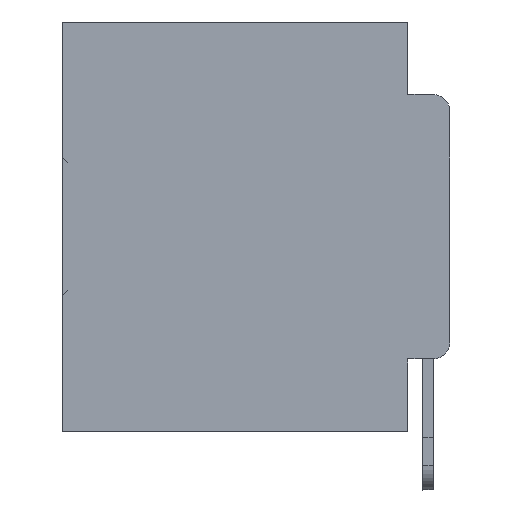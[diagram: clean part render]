
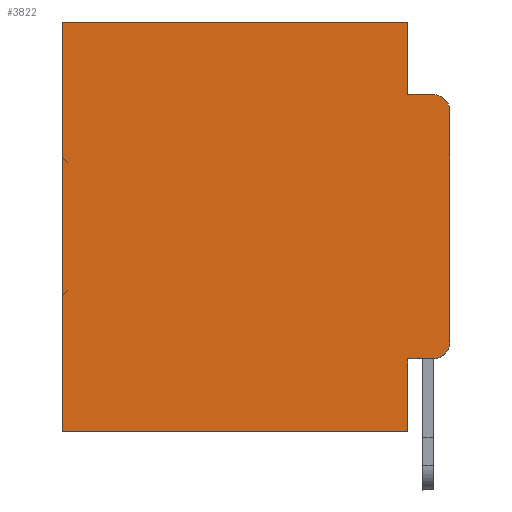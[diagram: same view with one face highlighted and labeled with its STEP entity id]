
A CAD part, left-side view. The second image highlights one B-rep face of the part: STEP entity #3822.
In plain terms, the highlighted planar face has unit normal (-1, 0, 0).
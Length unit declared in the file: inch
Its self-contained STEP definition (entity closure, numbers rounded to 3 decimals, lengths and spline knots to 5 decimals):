
#352 = VERTEX_POINT ( 'NONE', #25775 ) ;
#742 = ORIENTED_EDGE ( 'NONE', *, *, #15955, .T. ) ;
#1709 = EDGE_CURVE ( 'NONE', #17315, #6882, #31972, .T. ) ;
#2109 = FACE_OUTER_BOUND ( 'NONE', #27719, .T. ) ;
#2655 = CARTESIAN_POINT ( 'NONE',  ( 0.298, 0.051, -0.0885 ) ) ;
#2982 = DIRECTION ( 'NONE',  ( 0., 1., 0. ) ) ;
#3738 = EDGE_CURVE ( 'NONE', #15102, #352, #27232, .T. ) ;
#3822 = ADVANCED_FACE ( 'NONE', ( #2109 ), #8404, .F. ) ;
#3905 = LINE ( 'NONE', #7316, #31118 ) ;
#4172 = VERTEX_POINT ( 'NONE', #20966 ) ;
#4477 = CARTESIAN_POINT ( 'NONE',  ( 0.298, 0.02, -0.1085 ) ) ;
#4622 = CARTESIAN_POINT ( 'NONE',  ( 0.298, 0.473, 0. ) ) ;
#4858 = LINE ( 'NONE', #4622, #24842 ) ;
#5087 = CARTESIAN_POINT ( 'NONE',  ( 0.298, 0.02, -0.4115 ) ) ;
#6058 = LINE ( 'NONE', #23870, #23077 ) ;
#6618 = CARTESIAN_POINT ( 'NONE',  ( 0.298, 0.051, -0.0885 ) ) ;
#6882 = VERTEX_POINT ( 'NONE', #34267 ) ;
#6976 = EDGE_CURVE ( 'NONE', #32671, #15608, #25471, .T. ) ;
#7316 = CARTESIAN_POINT ( 'NONE',  ( 0.298, 0.051, 0. ) ) ;
#7762 = LINE ( 'NONE', #33624, #21792 ) ;
#8161 = ORIENTED_EDGE ( 'NONE', *, *, #6976, .T. ) ;
#8404 = PLANE ( 'NONE',  #27809 ) ;
#8769 = VERTEX_POINT ( 'NONE', #34031 ) ;
#9169 = ORIENTED_EDGE ( 'NONE', *, *, #22297, .F. ) ;
#9246 = DIRECTION ( 'NONE',  ( 0., -1., 0. ) ) ;
#9436 = CARTESIAN_POINT ( 'NONE',  ( 0.298, 0., -0.1085 ) ) ;
#10993 = CARTESIAN_POINT ( 'NONE',  ( 0.298, 0.051, -0.5 ) ) ;
#11136 = DIRECTION ( 'NONE',  ( 1., 0., 0. ) ) ;
#11978 = LINE ( 'NONE', #13156, #23455 ) ;
#12300 = ORIENTED_EDGE ( 'NONE', *, *, #1709, .T. ) ;
#12671 = VERTEX_POINT ( 'NONE', #10993 ) ;
#13156 = CARTESIAN_POINT ( 'NONE',  ( 0.298, 0., 0. ) ) ;
#13269 = ORIENTED_EDGE ( 'NONE', *, *, #22045, .T. ) ;
#13586 = CARTESIAN_POINT ( 'NONE',  ( 0.298, 0., -0.5 ) ) ;
#13804 = CARTESIAN_POINT ( 'NONE',  ( 0.298, 0.051, 0. ) ) ;
#15102 = VERTEX_POINT ( 'NONE', #5087 ) ;
#15574 = DIRECTION ( 'NONE',  ( 0., 0., -1. ) ) ;
#15599 = AXIS2_PLACEMENT_3D ( 'NONE', #4477, #23486, #26235 ) ;
#15608 = VERTEX_POINT ( 'NONE', #20099 ) ;
#15955 = EDGE_CURVE ( 'NONE', #6882, #4172, #4858, .T. ) ;
#16057 = LINE ( 'NONE', #6618, #27477 ) ;
#16277 = DIRECTION ( 'NONE',  ( 0., 0., -1. ) ) ;
#16452 = AXIS2_PLACEMENT_3D ( 'NONE', #32266, #24303, #16277 ) ;
#17315 = VERTEX_POINT ( 'NONE', #13804 ) ;
#17327 = DIRECTION ( 'NONE',  ( 0., 1., 0. ) ) ;
#20099 = CARTESIAN_POINT ( 'NONE',  ( 0.298, 0.02, -0.0885 ) ) ;
#20966 = CARTESIAN_POINT ( 'NONE',  ( 0.298, 0.473, -0.5 ) ) ;
#21792 = VECTOR ( 'NONE', #28279, 39.37008 ) ;
#22045 = EDGE_CURVE ( 'NONE', #8769, #15102, #7762, .T. ) ;
#22258 = ORIENTED_EDGE ( 'NONE', *, *, #3738, .T. ) ;
#22297 = EDGE_CURVE ( 'NONE', #8769, #12671, #6058, .T. ) ;
#22422 = DIRECTION ( 'NONE',  ( 0., 0., -1. ) ) ;
#22916 = EDGE_CURVE ( 'NONE', #32671, #352, #11978, .T. ) ;
#23077 = VECTOR ( 'NONE', #34887, 39.37008 ) ;
#23455 = VECTOR ( 'NONE', #32130, 39.37008 ) ;
#23486 = DIRECTION ( 'NONE',  ( -1., 0., 0. ) ) ;
#23870 = CARTESIAN_POINT ( 'NONE',  ( 0.298, 0.051, 0. ) ) ;
#23881 = LINE ( 'NONE', #13586, #31106 ) ;
#24303 = DIRECTION ( 'NONE',  ( -1., 0., 0. ) ) ;
#24517 = ORIENTED_EDGE ( 'NONE', *, *, #22916, .F. ) ;
#24570 = EDGE_CURVE ( 'NONE', #12671, #4172, #23881, .T. ) ;
#24842 = VECTOR ( 'NONE', #15574, 39.37008 ) ;
#25471 = CIRCLE ( 'NONE', #15599, 0.02 ) ;
#25775 = CARTESIAN_POINT ( 'NONE',  ( 0.298, 0., -0.3915 ) ) ;
#26235 = DIRECTION ( 'NONE',  ( 0., 0., -1. ) ) ;
#27232 = CIRCLE ( 'NONE', #16452, 0.02 ) ;
#27477 = VECTOR ( 'NONE', #9246, 39.37008 ) ;
#27719 = EDGE_LOOP ( 'NONE', ( #24517, #8161, #35073, #29919, #12300, #742, #34843, #9169, #13269, #22258 ) ) ;
#27809 = AXIS2_PLACEMENT_3D ( 'NONE', #32845, #11136, #22422 ) ;
#28165 = VECTOR ( 'NONE', #17327, 39.37008 ) ;
#28279 = DIRECTION ( 'NONE',  ( 0., -1., 0. ) ) ;
#29058 = DIRECTION ( 'NONE',  ( 0., 0., -1. ) ) ;
#29919 = ORIENTED_EDGE ( 'NONE', *, *, #30443, .F. ) ;
#30443 = EDGE_CURVE ( 'NONE', #17315, #33713, #3905, .T. ) ;
#31106 = VECTOR ( 'NONE', #2982, 39.37008 ) ;
#31118 = VECTOR ( 'NONE', #29058, 39.37008 ) ;
#31946 = EDGE_CURVE ( 'NONE', #33713, #15608, #16057, .T. ) ;
#31972 = LINE ( 'NONE', #33441, #28165 ) ;
#32130 = DIRECTION ( 'NONE',  ( 0., 0., -1. ) ) ;
#32266 = CARTESIAN_POINT ( 'NONE',  ( 0.298, 0.02, -0.3915 ) ) ;
#32671 = VERTEX_POINT ( 'NONE', #9436 ) ;
#32845 = CARTESIAN_POINT ( 'NONE',  ( 0.298, 0., 0. ) ) ;
#33441 = CARTESIAN_POINT ( 'NONE',  ( 0.298, 0., 0. ) ) ;
#33624 = CARTESIAN_POINT ( 'NONE',  ( 0.298, 0.051, -0.4115 ) ) ;
#33713 = VERTEX_POINT ( 'NONE', #2655 ) ;
#34031 = CARTESIAN_POINT ( 'NONE',  ( 0.298, 0.051, -0.4115 ) ) ;
#34267 = CARTESIAN_POINT ( 'NONE',  ( 0.298, 0.473, 0. ) ) ;
#34843 = ORIENTED_EDGE ( 'NONE', *, *, #24570, .F. ) ;
#34887 = DIRECTION ( 'NONE',  ( 0., 0., -1. ) ) ;
#35073 = ORIENTED_EDGE ( 'NONE', *, *, #31946, .F. ) ;
